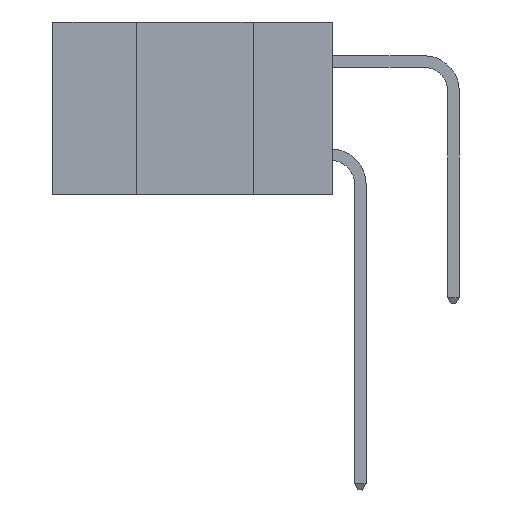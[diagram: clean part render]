
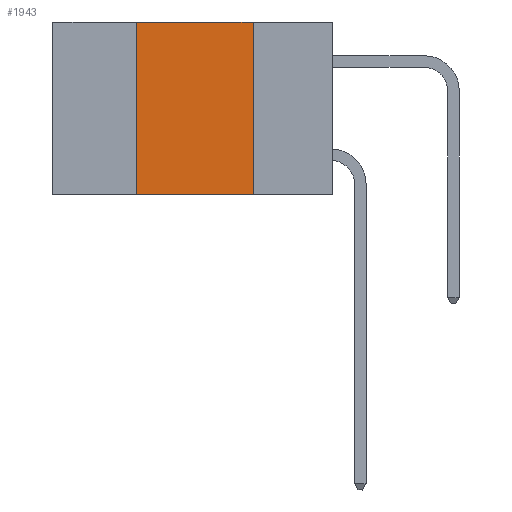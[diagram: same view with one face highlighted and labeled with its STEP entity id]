
A CAD part, left-side view. The second image highlights one B-rep face of the part: STEP entity #1943.
In plain terms, the highlighted planar face has unit normal (-1, 0, 0).
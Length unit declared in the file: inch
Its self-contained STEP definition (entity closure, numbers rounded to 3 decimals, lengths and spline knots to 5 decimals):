
#447 = AXIS2_PLACEMENT_3D ( 'NONE', #5589, #13526, #3156 ) ;
#738 = VERTEX_POINT ( 'NONE', #12308 ) ;
#1034 = CARTESIAN_POINT ( 'NONE',  ( 0., 0.42, 0. ) ) ;
#1077 = PLANE ( 'NONE',  #447 ) ;
#1672 = ORIENTED_EDGE ( 'NONE', *, *, #9373, .F. ) ;
#1943 = ADVANCED_FACE ( 'NONE', ( #11363 ), #1077, .F. ) ;
#2014 = CARTESIAN_POINT ( 'NONE',  ( 0., 0.42, -0.37 ) ) ;
#2262 = EDGE_CURVE ( 'NONE', #11268, #9470, #14621, .T. ) ;
#2421 = LINE ( 'NONE', #8973, #4200 ) ;
#3156 = DIRECTION ( 'NONE',  ( 0., 0., -1. ) ) ;
#4200 = VECTOR ( 'NONE', #6956, 39.37008 ) ;
#4683 = ORIENTED_EDGE ( 'NONE', *, *, #5814, .T. ) ;
#4700 = CARTESIAN_POINT ( 'NONE',  ( 0., 0.6, 0. ) ) ;
#5293 = ORIENTED_EDGE ( 'NONE', *, *, #2262, .F. ) ;
#5589 = CARTESIAN_POINT ( 'NONE',  ( 0., 0.6, 0. ) ) ;
#5814 = EDGE_CURVE ( 'NONE', #11268, #8579, #7155, .T. ) ;
#6537 = DIRECTION ( 'NONE',  ( 0., 0., 1. ) ) ;
#6956 = DIRECTION ( 'NONE',  ( 0., 0., -1. ) ) ;
#7155 = LINE ( 'NONE', #9238, #14632 ) ;
#8579 = VERTEX_POINT ( 'NONE', #13382 ) ;
#8699 = EDGE_CURVE ( 'NONE', #738, #8579, #2421, .T. ) ;
#8973 = CARTESIAN_POINT ( 'NONE',  ( 0., 0.17, -0.37 ) ) ;
#9174 = CARTESIAN_POINT ( 'NONE',  ( 0., 0.42, -0.37 ) ) ;
#9238 = CARTESIAN_POINT ( 'NONE',  ( 0., 0.6, -0.37 ) ) ;
#9252 = DIRECTION ( 'NONE',  ( 0., -1., 0. ) ) ;
#9373 = EDGE_CURVE ( 'NONE', #9470, #738, #14317, .T. ) ;
#9382 = DIRECTION ( 'NONE',  ( 0., -1., 0. ) ) ;
#9470 = VERTEX_POINT ( 'NONE', #1034 ) ;
#10271 = EDGE_LOOP ( 'NONE', ( #10625, #1672, #5293, #4683 ) ) ;
#10625 = ORIENTED_EDGE ( 'NONE', *, *, #8699, .F. ) ;
#10721 = VECTOR ( 'NONE', #9252, 39.37008 ) ;
#11268 = VERTEX_POINT ( 'NONE', #9174 ) ;
#11363 = FACE_OUTER_BOUND ( 'NONE', #10271, .T. ) ;
#11405 = VECTOR ( 'NONE', #6537, 39.37008 ) ;
#12308 = CARTESIAN_POINT ( 'NONE',  ( 0., 0.17, 0. ) ) ;
#13382 = CARTESIAN_POINT ( 'NONE',  ( 0., 0.17, -0.37 ) ) ;
#13526 = DIRECTION ( 'NONE',  ( 1., 0., 0. ) ) ;
#14317 = LINE ( 'NONE', #4700, #10721 ) ;
#14621 = LINE ( 'NONE', #2014, #11405 ) ;
#14632 = VECTOR ( 'NONE', #9382, 39.37008 ) ;
